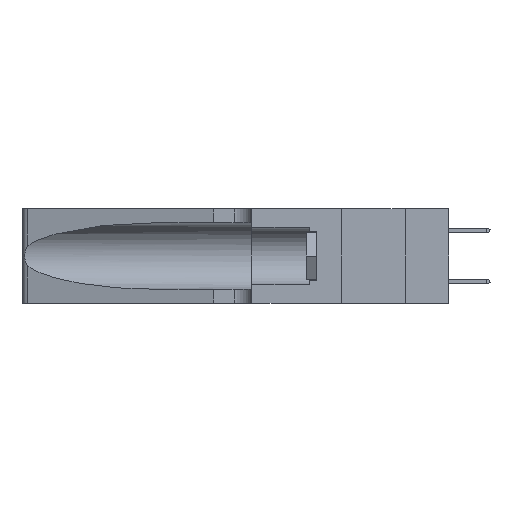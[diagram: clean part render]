
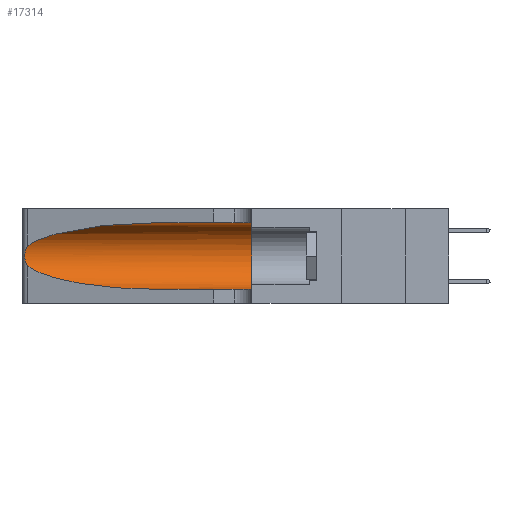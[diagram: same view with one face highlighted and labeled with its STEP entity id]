
A CAD part, left-side view. The second image highlights one B-rep face of the part: STEP entity #17314.
In plain terms, the highlighted cylindrical face has radius 3.308 mm (diameter 6.617 mm), a partial arc.
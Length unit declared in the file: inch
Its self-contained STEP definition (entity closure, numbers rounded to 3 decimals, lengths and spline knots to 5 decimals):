
#535 = CARTESIAN_POINT ( 'NONE',  ( 0.18966, 0.96281, 0.31525 ) ) ;
#718 = ORIENTED_EDGE ( 'NONE', *, *, #23428, .T. ) ;
#966 = VECTOR ( 'NONE', #3833, 39.37008 ) ;
#1125 = CARTESIAN_POINT ( 'NONE',  ( 0.1305, 0.72297, 0.05475 ) ) ;
#1482 = AXIS2_PLACEMENT_3D ( 'NONE', #9389, #23063, #11373 ) ;
#1801 = VERTEX_POINT ( 'NONE', #11631 ) ;
#3059 = VERTEX_POINT ( 'NONE', #23265 ) ;
#3461 = CARTESIAN_POINT ( 'NONE',  ( 0.25787, 1.23484, 0.2124 ) ) ;
#3553 = CARTESIAN_POINT ( 'NONE',  ( 0.1305, 1.61858, 0.185 ) ) ;
#3833 = DIRECTION ( 'NONE',  ( 0., -1., 0. ) ) ;
#4203 = EDGE_CURVE ( 'NONE', #15752, #7036, #24100, .T. ) ;
#5279 = VERTEX_POINT ( 'NONE', #9929 ) ;
#5482 = CARTESIAN_POINT ( 'NONE',  ( 0.26018, 1.23835, 0.19895 ) ) ;
#5842 = CYLINDRICAL_SURFACE ( 'NONE', #15717, 0.13025 ) ;
#6653 = CARTESIAN_POINT ( 'NONE',  ( 0.25487, 1.22718, 0.22369 ) ) ;
#6973 = LINE ( 'NONE', #19613, #966 ) ;
#7036 = VERTEX_POINT ( 'NONE', #11427 ) ;
#7087 = CARTESIAN_POINT ( 'NONE',  ( 0.25487, 1.22718, 0.14631 ) ) ;
#7100 = FACE_OUTER_BOUND ( 'NONE', #18725, .T. ) ;
#7505 = CARTESIAN_POINT ( 'NONE',  ( 0.26075, 1.23896, 0.178 ) ) ;
#9170 = EDGE_CURVE ( 'NONE', #3059, #14527, #15017, .T. ) ;
#9389 = CARTESIAN_POINT ( 'NONE',  ( 0.1305, 0.35, 0.185 ) ) ;
#9479 = CARTESIAN_POINT ( 'NONE',  ( 0.25856, 1.23593, 0.16098 ) ) ;
#9841 = DIRECTION ( 'NONE',  ( 0., -1., 0. ) ) ;
#9929 = CARTESIAN_POINT ( 'NONE',  ( 0.1305, 0.35, 0.05475 ) ) ;
#10922 = ORIENTED_EDGE ( 'NONE', *, *, #20489, .F. ) ;
#11084 = CARTESIAN_POINT ( 'NONE',  ( 0.2373, 1.15595, 0.08982 ) ) ;
#11373 = DIRECTION ( 'NONE',  ( 0., 0., 1. ) ) ;
#11379 = CARTESIAN_POINT ( 'NONE',  ( 0.25487, 1.22718, 0.22369 ) ) ;
#11427 = CARTESIAN_POINT ( 'NONE',  ( 0.1305, 0.72297, 0.05475 ) ) ;
#11466 = CARTESIAN_POINT ( 'NONE',  ( 0.25639, 1.23186, 0.15144 ) ) ;
#11631 = CARTESIAN_POINT ( 'NONE',  ( 0.1305, 0.35, 0.31525 ) ) ;
#11821 = ORIENTED_EDGE ( 'NONE', *, *, #13949, .F. ) ;
#12214 = LINE ( 'NONE', #21556, #22605 ) ;
#13046 = CARTESIAN_POINT ( 'NONE',  ( 0.18966, 0.96281, 0.05475 ) ) ;
#13142 = B_SPLINE_CURVE_WITH_KNOTS ( 'NONE', 3,
 ( #11379, #13322, #15282, #3461, #17285, #5482, #19277, #7505, #21187, #9479, #23155, #11466, #25101, #13417 ),
 .UNSPECIFIED., .F., .F.,
 ( 4, 2, 2, 2, 2, 2, 4 ),
 ( 0., 0.00027, 0.00053, 0.00107, 0.0016, 0.00187, 0.00214 ),
 .UNSPECIFIED. ) ;
#13164 = ORIENTED_EDGE ( 'NONE', *, *, #4203, .T. ) ;
#13322 = CARTESIAN_POINT ( 'NONE',  ( 0.25555, 1.22994, 0.2215 ) ) ;
#13417 = CARTESIAN_POINT ( 'NONE',  ( 0.25487, 1.22718, 0.14631 ) ) ;
#13949 = EDGE_CURVE ( 'NONE', #3059, #1801, #6973, .T. ) ;
#14444 = CARTESIAN_POINT ( 'NONE',  ( 0.1305, 0.72297, 0.31525 ) ) ;
#14527 = VERTEX_POINT ( 'NONE', #21259 ) ;
#15017 =( BOUNDED_CURVE ( )  B_SPLINE_CURVE ( 3, ( #14444, #535, #18435, #6653 ),
 .UNSPECIFIED., .F., .F. ) 
 B_SPLINE_CURVE_WITH_KNOTS ( ( 4, 4 ),
 ( 1.5708, 2.84003 ),
 .UNSPECIFIED. ) 
 CURVE ( )  GEOMETRIC_REPRESENTATION_ITEM ( )  RATIONAL_B_SPLINE_CURVE ( ( 1., 0.87, 0.87, 1. ) ) 
 REPRESENTATION_ITEM ( '' )  );
#15282 = CARTESIAN_POINT ( 'NONE',  ( 0.25639, 1.23184, 0.21858 ) ) ;
#15368 = DIRECTION ( 'NONE',  ( 0., 0., -1. ) ) ;
#15717 = AXIS2_PLACEMENT_3D ( 'NONE', #3553, #17376, #15368 ) ;
#15752 = VERTEX_POINT ( 'NONE', #7087 ) ;
#17285 = CARTESIAN_POINT ( 'NONE',  ( 0.25854, 1.2359, 0.20912 ) ) ;
#17314 = ADVANCED_FACE ( 'NONE', ( #7100 ), #5842, .F. ) ;
#17376 = DIRECTION ( 'NONE',  ( 0., -1., 0. ) ) ;
#17890 = ORIENTED_EDGE ( 'NONE', *, *, #22422, .T. ) ;
#18435 = CARTESIAN_POINT ( 'NONE',  ( 0.2373, 1.15595, 0.28018 ) ) ;
#18725 = EDGE_LOOP ( 'NONE', ( #24958, #17890, #13164, #718, #10922, #11821 ) ) ;
#19277 = CARTESIAN_POINT ( 'NONE',  ( 0.26075, 1.23896, 0.19203 ) ) ;
#19613 = CARTESIAN_POINT ( 'NONE',  ( 0.1305, 1.61858, 0.31525 ) ) ;
#20489 = EDGE_CURVE ( 'NONE', #1801, #5279, #21800, .T. ) ;
#21187 = CARTESIAN_POINT ( 'NONE',  ( 0.26017, 1.23833, 0.17102 ) ) ;
#21259 = CARTESIAN_POINT ( 'NONE',  ( 0.25487, 1.22718, 0.22369 ) ) ;
#21556 = CARTESIAN_POINT ( 'NONE',  ( 0.1305, 1.61858, 0.05475 ) ) ;
#21800 = CIRCLE ( 'NONE', #1482, 0.13025 ) ;
#22422 = EDGE_CURVE ( 'NONE', #14527, #15752, #13142, .T. ) ;
#22605 = VECTOR ( 'NONE', #9841, 39.37008 ) ;
#23063 = DIRECTION ( 'NONE',  ( 0., 1., 0. ) ) ;
#23155 = CARTESIAN_POINT ( 'NONE',  ( 0.25789, 1.23486, 0.15765 ) ) ;
#23265 = CARTESIAN_POINT ( 'NONE',  ( 0.1305, 0.72297, 0.31525 ) ) ;
#23428 = EDGE_CURVE ( 'NONE', #7036, #5279, #12214, .T. ) ;
#24100 =( BOUNDED_CURVE ( )  B_SPLINE_CURVE ( 3, ( #24742, #11084, #13046, #1125 ),
 .UNSPECIFIED., .F., .T. ) 
 B_SPLINE_CURVE_WITH_KNOTS ( ( 4, 4 ),
 ( 3.44316, 4.71239 ),
 .UNSPECIFIED. ) 
 CURVE ( )  GEOMETRIC_REPRESENTATION_ITEM ( )  RATIONAL_B_SPLINE_CURVE ( ( 1., 0.87, 0.87, 1. ) ) 
 REPRESENTATION_ITEM ( '' )  );
#24742 = CARTESIAN_POINT ( 'NONE',  ( 0.25487, 1.22718, 0.14631 ) ) ;
#24958 = ORIENTED_EDGE ( 'NONE', *, *, #9170, .T. ) ;
#25101 = CARTESIAN_POINT ( 'NONE',  ( 0.25555, 1.22993, 0.14849 ) ) ;
